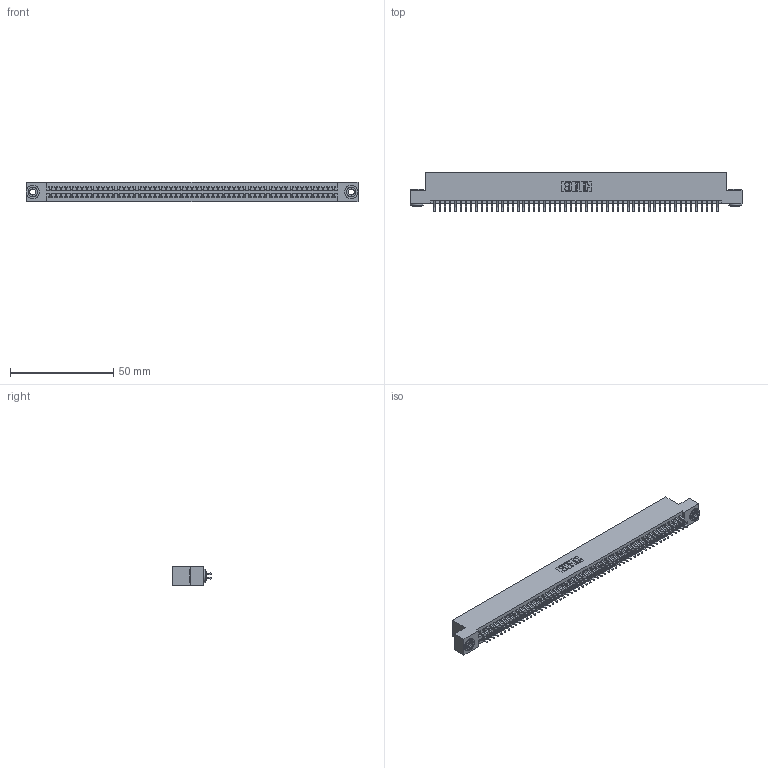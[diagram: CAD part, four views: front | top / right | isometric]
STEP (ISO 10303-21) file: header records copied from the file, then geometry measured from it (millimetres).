
FILE_DESCRIPTION (( 'STEP AP203' ), '1' );
FILE_NAME ('395-110-556-203.STEP', '2018-12-01T04:51:06', ( '' ), ( '' ), 'SwSTEP 2.0', 'SolidWorks 2016', '' );
FILE_SCHEMA (( 'CONFIG_CONTROL_DESIGN' ));
Length unit declared in the file: inch
Products named in the file (4): 395-110-556-203; 345-292-001_556 Tail; 345 Part_Flush Mounting Lugs - 0.156 Dia-TH; 345-250-002_345-250-002-102
Assembly tree (113 placements, depth 2):
  395-110-556-203
    345 Part_Flush Mounting Lugs - 0.156 Dia-TH
    345-292-001_556 Tail  x110
    345-250-002_345-250-002-102  x2
Bounding box: 160.91 x 19.24 x 9.4 mm (x, y, z)
Volume: 15766.6 mm3; surface area: 23666 mm2
Topology: 113 solids, 113 shells, 6324 faces, 18787 edges, 12374 vertices
Faces by surface type: plane 4160, cylinder 2156, cone 8
Entity records: 42274 total; most frequent: CARTESIAN_POINT 7063, ORIENTED_EDGE 6978, DIRECTION 6231, EDGE_CURVE 3489, LINE 3105, VECTOR 3105, VERTEX_POINT 2322, AXIS2_PLACEMENT_3D 1563
